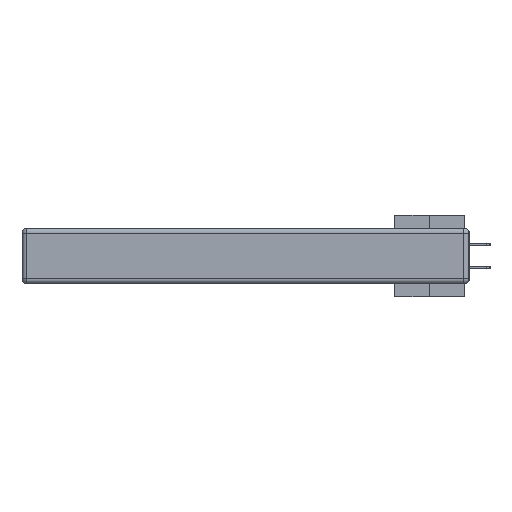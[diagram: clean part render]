
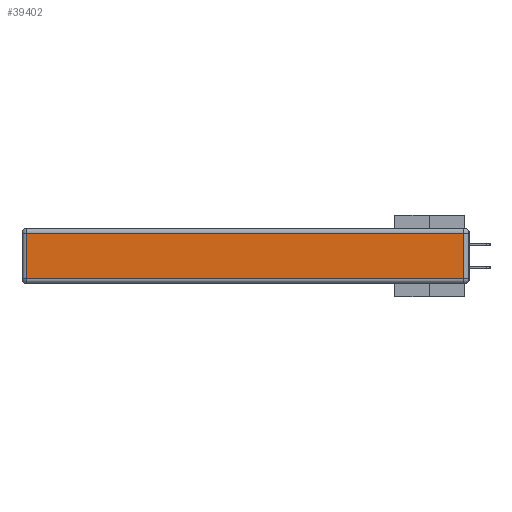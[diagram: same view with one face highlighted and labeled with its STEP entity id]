
A CAD part, left-side view. The second image highlights one B-rep face of the part: STEP entity #39402.
In plain terms, the highlighted planar face has unit normal (-1, 0, 0).
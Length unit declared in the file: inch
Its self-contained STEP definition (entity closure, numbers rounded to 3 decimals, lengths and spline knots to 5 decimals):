
#1596 = LINE ( 'NONE', #6881, #28924 ) ;
#5923 = ORIENTED_EDGE ( 'NONE', *, *, #39338, .T. ) ;
#6058 = CARTESIAN_POINT ( 'NONE',  ( 0., 2.72, -0.03 ) ) ;
#6881 = CARTESIAN_POINT ( 'NONE',  ( 0., 0., -0.313 ) ) ;
#7397 = EDGE_CURVE ( 'NONE', #19266, #33613, #47089, .T. ) ;
#9326 = CARTESIAN_POINT ( 'NONE',  ( 0., 0.03, -0.313 ) ) ;
#12857 = LINE ( 'NONE', #28214, #32262 ) ;
#13418 = CARTESIAN_POINT ( 'NONE',  ( 0., 0., -0.343 ) ) ;
#15344 = VERTEX_POINT ( 'NONE', #9326 ) ;
#18342 = VERTEX_POINT ( 'NONE', #28036 ) ;
#18884 = ORIENTED_EDGE ( 'NONE', *, *, #7397, .T. ) ;
#19266 = VERTEX_POINT ( 'NONE', #6058 ) ;
#20412 = PLANE ( 'NONE',  #25202 ) ;
#25202 = AXIS2_PLACEMENT_3D ( 'NONE', #13418, #46247, #31915 ) ;
#26536 = VECTOR ( 'NONE', #30429, 39.37008 ) ;
#27217 = CARTESIAN_POINT ( 'NONE',  ( 0., 2.72, -0.343 ) ) ;
#28036 = CARTESIAN_POINT ( 'NONE',  ( 0., 0.03, -0.03 ) ) ;
#28214 = CARTESIAN_POINT ( 'NONE',  ( 0., 2.75, -0.03 ) ) ;
#28924 = VECTOR ( 'NONE', #44280, 39.37008 ) ;
#29726 = ORIENTED_EDGE ( 'NONE', *, *, #38242, .T. ) ;
#30429 = DIRECTION ( 'NONE',  ( 0., 0., -1. ) ) ;
#30858 = ORIENTED_EDGE ( 'NONE', *, *, #44374, .T. ) ;
#31915 = DIRECTION ( 'NONE',  ( 0., 0., 1. ) ) ;
#32262 = VECTOR ( 'NONE', #46410, 39.37008 ) ;
#33613 = VERTEX_POINT ( 'NONE', #35003 ) ;
#33913 = EDGE_LOOP ( 'NONE', ( #29726, #30858, #5923, #18884 ) ) ;
#35003 = CARTESIAN_POINT ( 'NONE',  ( 0., 2.72, -0.313 ) ) ;
#35828 = CARTESIAN_POINT ( 'NONE',  ( 0., 0.03, -0.343 ) ) ;
#37492 = LINE ( 'NONE', #35828, #39755 ) ;
#38242 = EDGE_CURVE ( 'NONE', #33613, #15344, #1596, .T. ) ;
#39338 = EDGE_CURVE ( 'NONE', #18342, #19266, #12857, .T. ) ;
#39402 = ADVANCED_FACE ( 'NONE', ( #39611 ), #20412, .T. ) ;
#39611 = FACE_OUTER_BOUND ( 'NONE', #33913, .T. ) ;
#39755 = VECTOR ( 'NONE', #42689, 39.37008 ) ;
#42689 = DIRECTION ( 'NONE',  ( 0., 0., 1. ) ) ;
#44280 = DIRECTION ( 'NONE',  ( 0., -1., 0. ) ) ;
#44374 = EDGE_CURVE ( 'NONE', #15344, #18342, #37492, .T. ) ;
#46247 = DIRECTION ( 'NONE',  ( -1., 0., 0. ) ) ;
#46410 = DIRECTION ( 'NONE',  ( 0., 1., 0. ) ) ;
#47089 = LINE ( 'NONE', #27217, #26536 ) ;
